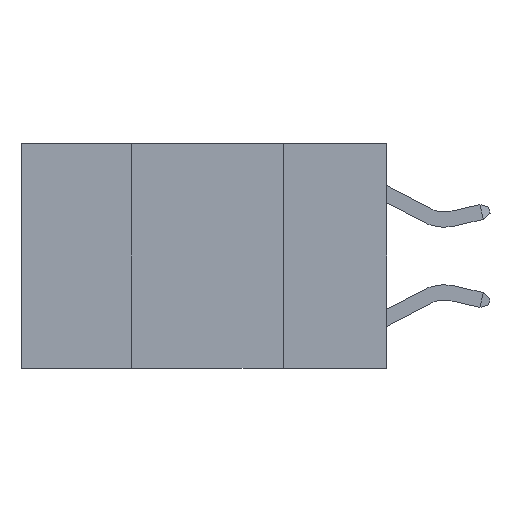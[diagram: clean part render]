
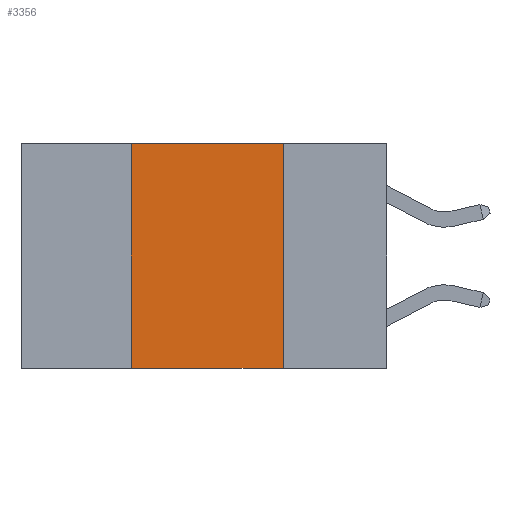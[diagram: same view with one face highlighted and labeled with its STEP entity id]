
A CAD part, left-side view. The second image highlights one B-rep face of the part: STEP entity #3356.
In plain terms, the highlighted planar face has unit normal (-1, 0, 0).
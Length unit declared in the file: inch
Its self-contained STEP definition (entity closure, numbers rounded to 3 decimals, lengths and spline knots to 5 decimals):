
#485 = CARTESIAN_POINT ( 'NONE',  ( 0., 0.42, -0.37 ) ) ;
#530 = LINE ( 'NONE', #1076, #2759 ) ;
#1076 = CARTESIAN_POINT ( 'NONE',  ( 0., 0.17, 0. ) ) ;
#2006 = DIRECTION ( 'NONE',  ( 0., 0., -1. ) ) ;
#2129 = CARTESIAN_POINT ( 'NONE',  ( 0., 0.6, 0. ) ) ;
#2234 = EDGE_CURVE ( 'NONE', #7691, #6384, #3372, .T. ) ;
#2540 = CARTESIAN_POINT ( 'NONE',  ( 0., 0.42, 0. ) ) ;
#2654 = EDGE_CURVE ( 'NONE', #3431, #5450, #530, .T. ) ;
#2759 = VECTOR ( 'NONE', #2006, 39.37008 ) ;
#3356 = ADVANCED_FACE ( 'NONE', ( #7817 ), #12070, .F. ) ;
#3372 = LINE ( 'NONE', #13015, #6930 ) ;
#3431 = VERTEX_POINT ( 'NONE', #6067 ) ;
#3838 = AXIS2_PLACEMENT_3D ( 'NONE', #5744, #5278, #4210 ) ;
#4210 = DIRECTION ( 'NONE',  ( 0., 0., -1. ) ) ;
#4500 = CARTESIAN_POINT ( 'NONE',  ( 0., 0.6, -0.37 ) ) ;
#4580 = EDGE_CURVE ( 'NONE', #6384, #3431, #6289, .T. ) ;
#5278 = DIRECTION ( 'NONE',  ( 1., 0., 0. ) ) ;
#5447 = ORIENTED_EDGE ( 'NONE', *, *, #4580, .F. ) ;
#5450 = VERTEX_POINT ( 'NONE', #12422 ) ;
#5744 = CARTESIAN_POINT ( 'NONE',  ( 0., 0.6, 0. ) ) ;
#6067 = CARTESIAN_POINT ( 'NONE',  ( 0., 0.17, 0. ) ) ;
#6289 = LINE ( 'NONE', #2129, #6975 ) ;
#6384 = VERTEX_POINT ( 'NONE', #2540 ) ;
#6930 = VECTOR ( 'NONE', #7812, 39.37008 ) ;
#6975 = VECTOR ( 'NONE', #12758, 39.37008 ) ;
#7691 = VERTEX_POINT ( 'NONE', #485 ) ;
#7812 = DIRECTION ( 'NONE',  ( 0., 0., 1. ) ) ;
#7817 = FACE_OUTER_BOUND ( 'NONE', #9382, .T. ) ;
#8230 = EDGE_CURVE ( 'NONE', #7691, #5450, #12166, .T. ) ;
#8755 = DIRECTION ( 'NONE',  ( 0., -1., 0. ) ) ;
#9382 = EDGE_LOOP ( 'NONE', ( #12958, #5447, #11709, #10437 ) ) ;
#10437 = ORIENTED_EDGE ( 'NONE', *, *, #8230, .T. ) ;
#11709 = ORIENTED_EDGE ( 'NONE', *, *, #2234, .F. ) ;
#12070 = PLANE ( 'NONE',  #3838 ) ;
#12166 = LINE ( 'NONE', #4500, #12323 ) ;
#12323 = VECTOR ( 'NONE', #8755, 39.37008 ) ;
#12422 = CARTESIAN_POINT ( 'NONE',  ( 0., 0.17, -0.37 ) ) ;
#12758 = DIRECTION ( 'NONE',  ( 0., -1., 0. ) ) ;
#12958 = ORIENTED_EDGE ( 'NONE', *, *, #2654, .F. ) ;
#13015 = CARTESIAN_POINT ( 'NONE',  ( 0., 0.42, 0. ) ) ;
